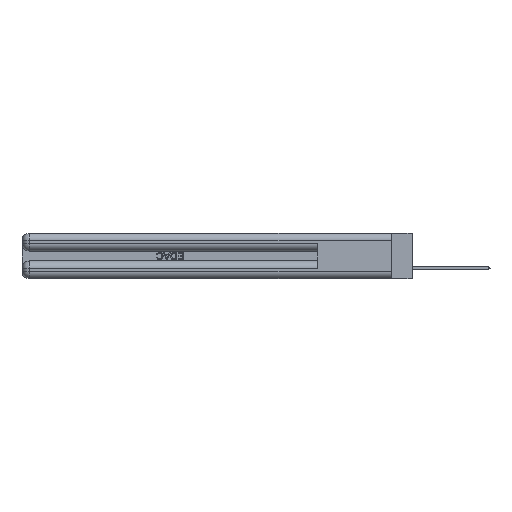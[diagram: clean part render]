
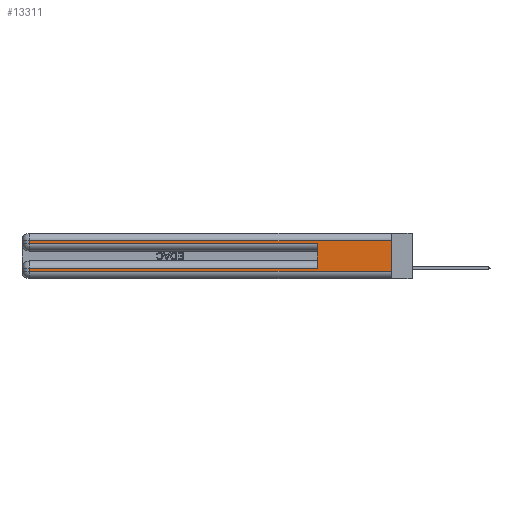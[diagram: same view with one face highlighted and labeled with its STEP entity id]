
A CAD part, left-side view. The second image highlights one B-rep face of the part: STEP entity #13311.
In plain terms, the highlighted planar face has unit normal (-1, 0, 0).
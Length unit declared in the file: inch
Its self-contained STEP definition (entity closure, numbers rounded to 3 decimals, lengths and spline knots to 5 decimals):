
#847 = CARTESIAN_POINT ( 'NONE',  ( 0., 0., 0.06 ) ) ;
#964 = ORIENTED_EDGE ( 'NONE', *, *, #20074, .T. ) ;
#1652 = CARTESIAN_POINT ( 'NONE',  ( 0., 2.94, 0.085 ) ) ;
#2079 = DIRECTION ( 'NONE',  ( 0., 0., -1. ) ) ;
#3578 = VECTOR ( 'NONE', #44742, 39.37008 ) ;
#3976 = EDGE_CURVE ( 'NONE', #6303, #43230, #17476, .T. ) ;
#4466 = EDGE_LOOP ( 'NONE', ( #5286, #4738, #16881, #44768, #42775, #11489, #26490, #964 ) ) ;
#4738 = ORIENTED_EDGE ( 'NONE', *, *, #48828, .T. ) ;
#5236 = AXIS2_PLACEMENT_3D ( 'NONE', #22947, #6559, #42176 ) ;
#5286 = ORIENTED_EDGE ( 'NONE', *, *, #14080, .F. ) ;
#5829 = FACE_OUTER_BOUND ( 'NONE', #4466, .T. ) ;
#5830 = DIRECTION ( 'NONE',  ( 0., -1., 0. ) ) ;
#6239 = VERTEX_POINT ( 'NONE', #1652 ) ;
#6303 = VERTEX_POINT ( 'NONE', #16658 ) ;
#6559 = DIRECTION ( 'NONE',  ( 1., 0., 0. ) ) ;
#7854 = VECTOR ( 'NONE', #5830, 39.37008 ) ;
#8774 = CARTESIAN_POINT ( 'NONE',  ( 0., 0.6, 0.145 ) ) ;
#9911 = VECTOR ( 'NONE', #21258, 39.37008 ) ;
#10096 = VERTEX_POINT ( 'NONE', #36222 ) ;
#11489 = ORIENTED_EDGE ( 'NONE', *, *, #17727, .T. ) ;
#11903 = CARTESIAN_POINT ( 'NONE',  ( 0., 2.94, 0.37 ) ) ;
#13311 = ADVANCED_FACE ( 'NONE', ( #5829 ), #19692, .F. ) ;
#14080 = EDGE_CURVE ( 'NONE', #27622, #14189, #49226, .T. ) ;
#14189 = VERTEX_POINT ( 'NONE', #42131 ) ;
#14439 = VERTEX_POINT ( 'NONE', #34551 ) ;
#15141 = LINE ( 'NONE', #45039, #7854 ) ;
#16027 = VERTEX_POINT ( 'NONE', #27152 ) ;
#16658 = CARTESIAN_POINT ( 'NONE',  ( 0., 2.94, 0.31 ) ) ;
#16881 = ORIENTED_EDGE ( 'NONE', *, *, #3976, .T. ) ;
#17476 = LINE ( 'NONE', #11903, #3578 ) ;
#17727 = EDGE_CURVE ( 'NONE', #14439, #6239, #23021, .T. ) ;
#17911 = CARTESIAN_POINT ( 'NONE',  ( 0., 0., 0.31 ) ) ;
#18211 = VECTOR ( 'NONE', #48988, 39.37008 ) ;
#19209 = VECTOR ( 'NONE', #26405, 39.37008 ) ;
#19692 = PLANE ( 'NONE',  #5236 ) ;
#19796 = LINE ( 'NONE', #8774, #27640 ) ;
#20074 = EDGE_CURVE ( 'NONE', #16027, #14189, #46946, .T. ) ;
#20762 = DIRECTION ( 'NONE',  ( 0., 0., 1. ) ) ;
#20920 = LINE ( 'NONE', #28256, #37351 ) ;
#21258 = DIRECTION ( 'NONE',  ( 0., 1., 0. ) ) ;
#22947 = CARTESIAN_POINT ( 'NONE',  ( 0., 0., 0.37 ) ) ;
#23021 = LINE ( 'NONE', #34029, #18211 ) ;
#24777 = EDGE_CURVE ( 'NONE', #6239, #16027, #20920, .T. ) ;
#26405 = DIRECTION ( 'NONE',  ( 0., -1., 0. ) ) ;
#26490 = ORIENTED_EDGE ( 'NONE', *, *, #24777, .T. ) ;
#27152 = CARTESIAN_POINT ( 'NONE',  ( 0., 2.94, 0.06 ) ) ;
#27622 = VERTEX_POINT ( 'NONE', #39177 ) ;
#27640 = VECTOR ( 'NONE', #20762, 39.37008 ) ;
#28084 = DIRECTION ( 'NONE',  ( 0., 0., -1. ) ) ;
#28256 = CARTESIAN_POINT ( 'NONE',  ( 0., 2.94, 0.37 ) ) ;
#32830 = EDGE_CURVE ( 'NONE', #43230, #10096, #15141, .T. ) ;
#34029 = CARTESIAN_POINT ( 'NONE',  ( 0., 0., 0.085 ) ) ;
#34551 = CARTESIAN_POINT ( 'NONE',  ( 0., 0.6, 0.085 ) ) ;
#36222 = CARTESIAN_POINT ( 'NONE',  ( 0., 0.6, 0.285 ) ) ;
#37246 = VECTOR ( 'NONE', #2079, 39.37008 ) ;
#37351 = VECTOR ( 'NONE', #28084, 39.37008 ) ;
#39177 = CARTESIAN_POINT ( 'NONE',  ( 0., 0., 0.31 ) ) ;
#42131 = CARTESIAN_POINT ( 'NONE',  ( 0., 0., 0.06 ) ) ;
#42176 = DIRECTION ( 'NONE',  ( 0., 0., -1. ) ) ;
#42775 = ORIENTED_EDGE ( 'NONE', *, *, #45080, .F. ) ;
#43230 = VERTEX_POINT ( 'NONE', #44672 ) ;
#44672 = CARTESIAN_POINT ( 'NONE',  ( 0., 2.94, 0.285 ) ) ;
#44742 = DIRECTION ( 'NONE',  ( 0., 0., -1. ) ) ;
#44768 = ORIENTED_EDGE ( 'NONE', *, *, #32830, .T. ) ;
#45039 = CARTESIAN_POINT ( 'NONE',  ( 0., 0., 0.285 ) ) ;
#45080 = EDGE_CURVE ( 'NONE', #14439, #10096, #19796, .T. ) ;
#46733 = LINE ( 'NONE', #17911, #9911 ) ;
#46946 = LINE ( 'NONE', #847, #19209 ) ;
#48335 = CARTESIAN_POINT ( 'NONE',  ( 0., 0., 0.37 ) ) ;
#48828 = EDGE_CURVE ( 'NONE', #27622, #6303, #46733, .T. ) ;
#48988 = DIRECTION ( 'NONE',  ( 0., 1., 0. ) ) ;
#49226 = LINE ( 'NONE', #48335, #37246 ) ;
